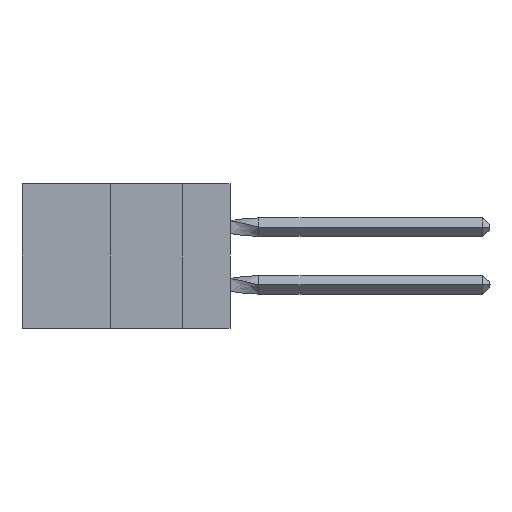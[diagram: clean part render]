
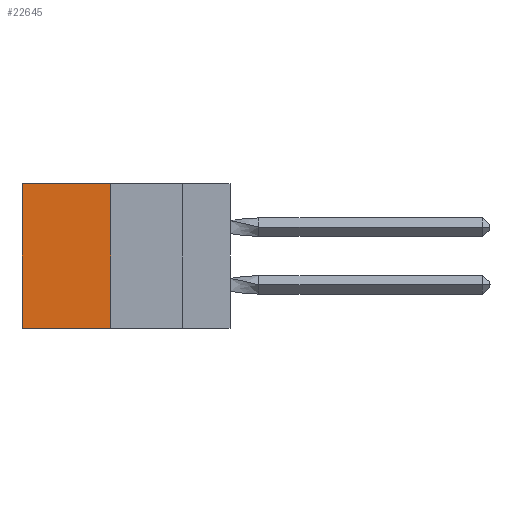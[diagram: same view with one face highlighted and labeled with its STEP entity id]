
A CAD part, left-side view. The second image highlights one B-rep face of the part: STEP entity #22645.
In plain terms, the highlighted planar face has unit normal (-1, 0, 0).
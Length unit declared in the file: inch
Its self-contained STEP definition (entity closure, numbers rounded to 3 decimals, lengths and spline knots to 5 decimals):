
#399 = CARTESIAN_POINT ( 'NONE',  ( 0.305, 0.72, -0.5 ) ) ;
#673 = FACE_OUTER_BOUND ( 'NONE', #11783, .T. ) ;
#1027 = CARTESIAN_POINT ( 'NONE',  ( 0.305, 0.413, 0. ) ) ;
#1285 = VERTEX_POINT ( 'NONE', #16257 ) ;
#2833 = DIRECTION ( 'NONE',  ( 0., 1., 0. ) ) ;
#3820 = CARTESIAN_POINT ( 'NONE',  ( 0.305, 0.413, -0.5 ) ) ;
#4655 = ORIENTED_EDGE ( 'NONE', *, *, #20437, .T. ) ;
#6404 = VECTOR ( 'NONE', #2833, 39.37008 ) ;
#6483 = VECTOR ( 'NONE', #18248, 39.37008 ) ;
#8165 = AXIS2_PLACEMENT_3D ( 'NONE', #3820, #13053, #16982 ) ;
#10319 = VERTEX_POINT ( 'NONE', #16511 ) ;
#11783 = EDGE_LOOP ( 'NONE', ( #4655, #21483, #16726, #14061 ) ) ;
#12056 = EDGE_CURVE ( 'NONE', #1285, #20928, #16357, .T. ) ;
#13053 = DIRECTION ( 'NONE',  ( 1., 0., 0. ) ) ;
#13451 = DIRECTION ( 'NONE',  ( 0., 0., -1. ) ) ;
#14061 = ORIENTED_EDGE ( 'NONE', *, *, #17782, .T. ) ;
#14797 = LINE ( 'NONE', #15417, #19181 ) ;
#15108 = PLANE ( 'NONE',  #8165 ) ;
#15417 = CARTESIAN_POINT ( 'NONE',  ( 0.305, 0.413, -0.5 ) ) ;
#16146 = CARTESIAN_POINT ( 'NONE',  ( 0.305, 0.413, -0.5 ) ) ;
#16257 = CARTESIAN_POINT ( 'NONE',  ( 0.305, 0.413, -0.5 ) ) ;
#16357 = LINE ( 'NONE', #16146, #6483 ) ;
#16511 = CARTESIAN_POINT ( 'NONE',  ( 0.305, 0.72, 0. ) ) ;
#16726 = ORIENTED_EDGE ( 'NONE', *, *, #20488, .F. ) ;
#16844 = VECTOR ( 'NONE', #17438, 39.37008 ) ;
#16982 = DIRECTION ( 'NONE',  ( 0., 0., -1. ) ) ;
#17327 = CARTESIAN_POINT ( 'NONE',  ( 0.305, 0.72, -0.5 ) ) ;
#17438 = DIRECTION ( 'NONE',  ( 0., 0., -1. ) ) ;
#17782 = EDGE_CURVE ( 'NONE', #18266, #10319, #23535, .T. ) ;
#18248 = DIRECTION ( 'NONE',  ( 0., 1., 0. ) ) ;
#18266 = VERTEX_POINT ( 'NONE', #1027 ) ;
#19181 = VECTOR ( 'NONE', #13451, 39.37008 ) ;
#19505 = CARTESIAN_POINT ( 'NONE',  ( 0.305, 0.413, 0. ) ) ;
#20437 = EDGE_CURVE ( 'NONE', #10319, #20928, #21774, .T. ) ;
#20488 = EDGE_CURVE ( 'NONE', #18266, #1285, #14797, .T. ) ;
#20928 = VERTEX_POINT ( 'NONE', #17327 ) ;
#21483 = ORIENTED_EDGE ( 'NONE', *, *, #12056, .F. ) ;
#21774 = LINE ( 'NONE', #399, #16844 ) ;
#22645 = ADVANCED_FACE ( 'NONE', ( #673 ), #15108, .F. ) ;
#23535 = LINE ( 'NONE', #19505, #6404 ) ;
